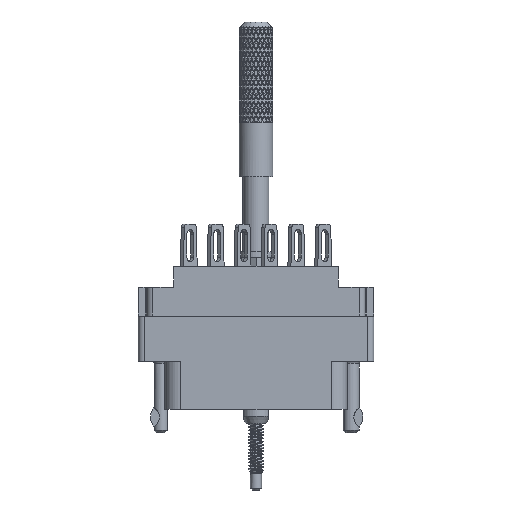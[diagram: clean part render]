
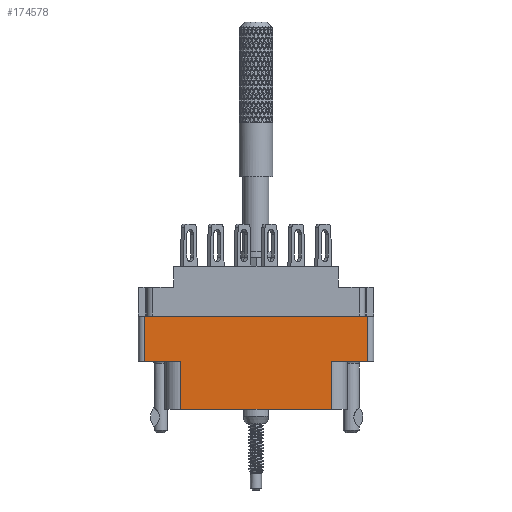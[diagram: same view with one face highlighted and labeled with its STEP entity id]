
A CAD part, front view. The second image highlights one B-rep face of the part: STEP entity #174578.
In plain terms, the highlighted planar face has unit normal (0, -1, 0).
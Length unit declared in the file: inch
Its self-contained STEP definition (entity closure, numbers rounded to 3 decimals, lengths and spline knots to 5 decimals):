
#990 = CARTESIAN_POINT ( 'NONE',  ( -0.42, -0.343, -0.529 ) ) ;
#1620 = ORIENTED_EDGE ( 'NONE', *, *, #181576, .T. ) ;
#2207 = LINE ( 'NONE', #153847, #34780 ) ;
#2590 = LINE ( 'NONE', #34971, #154093 ) ;
#8802 = CARTESIAN_POINT ( 'NONE',  ( 0.42, -0.343, -0.529 ) ) ;
#18705 = ORIENTED_EDGE ( 'NONE', *, *, #166111, .T. ) ;
#34780 = VECTOR ( 'NONE', #79585, 39.37008 ) ;
#34971 = CARTESIAN_POINT ( 'NONE',  ( -0.42, -0.343, -0.529 ) ) ;
#37792 = ORIENTED_EDGE ( 'NONE', *, *, #41654, .T. ) ;
#39890 = ORIENTED_EDGE ( 'NONE', *, *, #129888, .F. ) ;
#41091 = LINE ( 'NONE', #50666, #166720 ) ;
#41636 = DIRECTION ( 'NONE',  ( 1., 0., 0. ) ) ;
#41654 = EDGE_CURVE ( 'NONE', #93659, #134753, #172165, .T. ) ;
#48640 = EDGE_CURVE ( 'NONE', #128475, #54557, #171431, .T. ) ;
#50666 = CARTESIAN_POINT ( 'NONE',  ( 0.624, -0.343, -0.798 ) ) ;
#51107 = DIRECTION ( 'NONE',  ( 0., 0., -1. ) ) ;
#52474 = VECTOR ( 'NONE', #132128, 39.37008 ) ;
#54557 = VERTEX_POINT ( 'NONE', #111372 ) ;
#55430 = CARTESIAN_POINT ( 'NONE',  ( 0.624, -0.343, -0.529 ) ) ;
#60693 = DIRECTION ( 'NONE',  ( -1., 0., 0. ) ) ;
#65054 = DIRECTION ( 'NONE',  ( 0., 0., 1. ) ) ;
#69925 = VECTOR ( 'NONE', #60693, 39.37008 ) ;
#78053 = DIRECTION ( 'NONE',  ( 0., 0., -1. ) ) ;
#78989 = VERTEX_POINT ( 'NONE', #146615 ) ;
#79585 = DIRECTION ( 'NONE',  ( 0., 0., 1. ) ) ;
#79598 = EDGE_CURVE ( 'NONE', #93659, #128475, #2207, .T. ) ;
#84388 = VECTOR ( 'NONE', #51107, 39.37008 ) ;
#89803 = ORIENTED_EDGE ( 'NONE', *, *, #79598, .F. ) ;
#92751 = CARTESIAN_POINT ( 'NONE',  ( -0.624, -0.343, -0.798 ) ) ;
#93659 = VERTEX_POINT ( 'NONE', #133392 ) ;
#95951 = DIRECTION ( 'NONE',  ( 0., 0., -1. ) ) ;
#109854 = LINE ( 'NONE', #92751, #170333 ) ;
#111372 = CARTESIAN_POINT ( 'NONE',  ( 0.624, -0.343, -0.277 ) ) ;
#112267 = CARTESIAN_POINT ( 'NONE',  ( 0.42, -0.343, -0.529 ) ) ;
#119063 = LINE ( 'NONE', #148735, #69925 ) ;
#120449 = ORIENTED_EDGE ( 'NONE', *, *, #167072, .F. ) ;
#121387 = CARTESIAN_POINT ( 'NONE',  ( -0.42, -0.343, -0.798 ) ) ;
#122846 = VERTEX_POINT ( 'NONE', #121387 ) ;
#128475 = VERTEX_POINT ( 'NONE', #145552 ) ;
#129888 = EDGE_CURVE ( 'NONE', #174647, #78989, #144937, .T. ) ;
#131506 = CARTESIAN_POINT ( 'NONE',  ( -0.656, -0.343, -0.277 ) ) ;
#132128 = DIRECTION ( 'NONE',  ( 1., 0., 0. ) ) ;
#132853 = AXIS2_PLACEMENT_3D ( 'NONE', #168251, #170148, #95951 ) ;
#133392 = CARTESIAN_POINT ( 'NONE',  ( -0.624, -0.343, -0.529 ) ) ;
#134753 = VERTEX_POINT ( 'NONE', #990 ) ;
#136985 = VERTEX_POINT ( 'NONE', #55430 ) ;
#142457 = EDGE_CURVE ( 'NONE', #134753, #122846, #2590, .T. ) ;
#144937 = LINE ( 'NONE', #8802, #84388 ) ;
#145552 = CARTESIAN_POINT ( 'NONE',  ( -0.624, -0.343, -0.277 ) ) ;
#146333 = EDGE_LOOP ( 'NONE', ( #168598, #18705, #39890, #120449, #1620, #190410, #89803, #37792 ) ) ;
#146615 = CARTESIAN_POINT ( 'NONE',  ( 0.42, -0.343, -0.798 ) ) ;
#148735 = CARTESIAN_POINT ( 'NONE',  ( 0., -0.343, -0.529 ) ) ;
#153300 = DIRECTION ( 'NONE',  ( 1., 0., 0. ) ) ;
#153847 = CARTESIAN_POINT ( 'NONE',  ( -0.624, -0.343, -0.798 ) ) ;
#154093 = VECTOR ( 'NONE', #78053, 39.37008 ) ;
#155155 = PLANE ( 'NONE',  #132853 ) ;
#160285 = CARTESIAN_POINT ( 'NONE',  ( 0., -0.343, -0.529 ) ) ;
#162754 = VECTOR ( 'NONE', #41636, 39.37008 ) ;
#166111 = EDGE_CURVE ( 'NONE', #122846, #78989, #109854, .T. ) ;
#166720 = VECTOR ( 'NONE', #65054, 39.37008 ) ;
#167072 = EDGE_CURVE ( 'NONE', #136985, #174647, #119063, .T. ) ;
#168251 = CARTESIAN_POINT ( 'NONE',  ( -0.624, -0.343, -0.798 ) ) ;
#168598 = ORIENTED_EDGE ( 'NONE', *, *, #142457, .T. ) ;
#170148 = DIRECTION ( 'NONE',  ( 0., -1., 0. ) ) ;
#170333 = VECTOR ( 'NONE', #153300, 39.37008 ) ;
#171431 = LINE ( 'NONE', #131506, #52474 ) ;
#172165 = LINE ( 'NONE', #160285, #162754 ) ;
#174578 = ADVANCED_FACE ( 'NONE', ( #190958 ), #155155, .T. ) ;
#174647 = VERTEX_POINT ( 'NONE', #112267 ) ;
#181576 = EDGE_CURVE ( 'NONE', #136985, #54557, #41091, .T. ) ;
#190410 = ORIENTED_EDGE ( 'NONE', *, *, #48640, .F. ) ;
#190958 = FACE_OUTER_BOUND ( 'NONE', #146333, .T. ) ;
